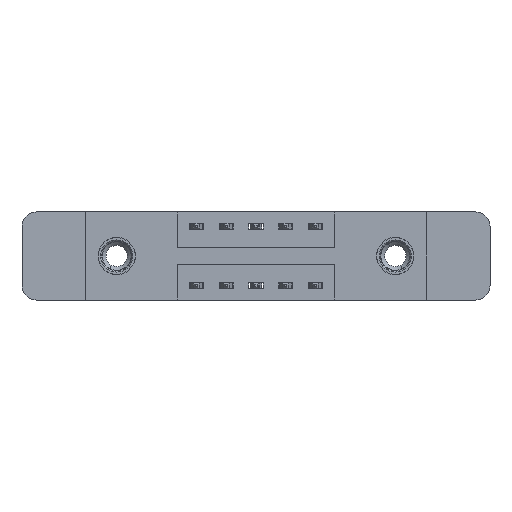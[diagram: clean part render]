
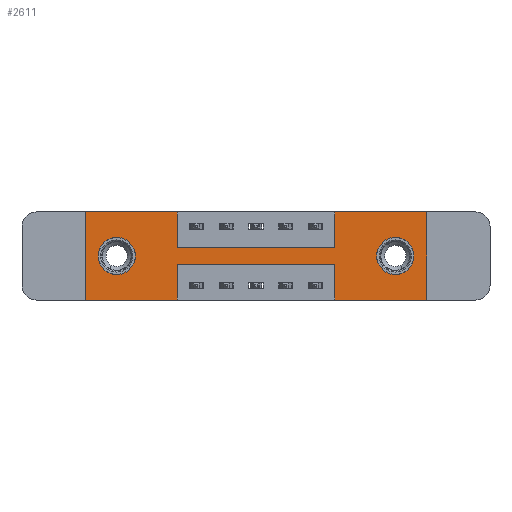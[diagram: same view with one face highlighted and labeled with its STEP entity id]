
A CAD part, front view. The second image highlights one B-rep face of the part: STEP entity #2611.
In plain terms, the highlighted planar face has unit normal (0, -1, 0).
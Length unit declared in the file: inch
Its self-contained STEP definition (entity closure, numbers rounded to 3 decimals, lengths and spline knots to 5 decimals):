
#114 = CARTESIAN_POINT ( 'NONE',  ( 1.0475, 0., 0. ) ) ;
#251 = CIRCLE ( 'NONE', #4269, 0.078 ) ;
#421 = VERTEX_POINT ( 'NONE', #11232 ) ;
#464 = EDGE_LOOP ( 'NONE', ( #4634, #6377, #11064, #1808, #10592, #12197, #609, #7411, #11130, #10439, #12892, #6052 ) ) ;
#492 = AXIS2_PLACEMENT_3D ( 'NONE', #10237, #594, #2548 ) ;
#591 = CARTESIAN_POINT ( 'NONE',  ( 1.3025, 0., -0.185 ) ) ;
#594 = DIRECTION ( 'NONE',  ( 0., 1., 0. ) ) ;
#609 = ORIENTED_EDGE ( 'NONE', *, *, #4410, .F. ) ;
#617 = VECTOR ( 'NONE', #7813, 39.37008 ) ;
#828 = CARTESIAN_POINT ( 'NONE',  ( 1.0475, 0., 0. ) ) ;
#1084 = VERTEX_POINT ( 'NONE', #4495 ) ;
#1183 = DIRECTION ( 'NONE',  ( 0., 0., -1. ) ) ;
#1267 = VECTOR ( 'NONE', #8334, 39.37008 ) ;
#1575 = DIRECTION ( 'NONE',  ( 0., 1., 0. ) ) ;
#1769 = VECTOR ( 'NONE', #8291, 39.37008 ) ;
#1782 = CARTESIAN_POINT ( 'NONE',  ( 0., 0., 0. ) ) ;
#1808 = ORIENTED_EDGE ( 'NONE', *, *, #2719, .F. ) ;
#1887 = VERTEX_POINT ( 'NONE', #10619 ) ;
#1908 = EDGE_CURVE ( 'NONE', #3533, #421, #5184, .T. ) ;
#1961 = CARTESIAN_POINT ( 'NONE',  ( 0., 0., 0. ) ) ;
#2085 = CARTESIAN_POINT ( 'NONE',  ( 0.3875, 0., -0.22 ) ) ;
#2548 = DIRECTION ( 'NONE',  ( 0., 0., -1. ) ) ;
#2595 = FACE_BOUND ( 'NONE', #10058, .T. ) ;
#2611 = ADVANCED_FACE ( 'NONE', ( #5841, #2595, #8096 ), #9073, .T. ) ;
#2719 = EDGE_CURVE ( 'NONE', #1887, #12294, #10290, .T. ) ;
#2818 = VECTOR ( 'NONE', #5249, 39.37008 ) ;
#2833 = DIRECTION ( 'NONE',  ( 1., 0., 0. ) ) ;
#3062 = VERTEX_POINT ( 'NONE', #9270 ) ;
#3256 = CIRCLE ( 'NONE', #3486, 0.078 ) ;
#3486 = AXIS2_PLACEMENT_3D ( 'NONE', #9402, #10741, #7279 ) ;
#3509 = EDGE_CURVE ( 'NONE', #6834, #1887, #9177, .T. ) ;
#3533 = VERTEX_POINT ( 'NONE', #4042 ) ;
#3568 = LINE ( 'NONE', #10120, #11354 ) ;
#3586 = CARTESIAN_POINT ( 'NONE',  ( 0., 0., -0.37 ) ) ;
#3628 = CARTESIAN_POINT ( 'NONE',  ( 1.435, 0., 0. ) ) ;
#3706 = VECTOR ( 'NONE', #5077, 39.37008 ) ;
#3946 = VERTEX_POINT ( 'NONE', #11497 ) ;
#4042 = CARTESIAN_POINT ( 'NONE',  ( 0., 0., 0. ) ) ;
#4269 = AXIS2_PLACEMENT_3D ( 'NONE', #12480, #6275, #10357 ) ;
#4318 = VERTEX_POINT ( 'NONE', #4919 ) ;
#4410 = EDGE_CURVE ( 'NONE', #7584, #10257, #6044, .T. ) ;
#4495 = CARTESIAN_POINT ( 'NONE',  ( 0.1325, 0., -0.263 ) ) ;
#4504 = CARTESIAN_POINT ( 'NONE',  ( 0., 0., -0.37 ) ) ;
#4634 = ORIENTED_EDGE ( 'NONE', *, *, #8993, .F. ) ;
#4919 = CARTESIAN_POINT ( 'NONE',  ( 0.1325, 0., -0.107 ) ) ;
#5027 = CARTESIAN_POINT ( 'NONE',  ( 0.3875, 0., -0.15 ) ) ;
#5077 = DIRECTION ( 'NONE',  ( -1., 0., 0. ) ) ;
#5184 = LINE ( 'NONE', #1961, #2818 ) ;
#5249 = DIRECTION ( 'NONE',  ( 1., 0., 0. ) ) ;
#5359 = ORIENTED_EDGE ( 'NONE', *, *, #10028, .T. ) ;
#5434 = VECTOR ( 'NONE', #2833, 39.37008 ) ;
#5790 = VERTEX_POINT ( 'NONE', #10631 ) ;
#5841 = FACE_BOUND ( 'NONE', #7109, .T. ) ;
#6044 = LINE ( 'NONE', #828, #6667 ) ;
#6052 = ORIENTED_EDGE ( 'NONE', *, *, #12785, .F. ) ;
#6210 = DIRECTION ( 'NONE',  ( 1., 0., 0. ) ) ;
#6275 = DIRECTION ( 'NONE',  ( 0., 1., 0. ) ) ;
#6377 = ORIENTED_EDGE ( 'NONE', *, *, #8666, .F. ) ;
#6405 = CIRCLE ( 'NONE', #9101, 0.078 ) ;
#6555 = CIRCLE ( 'NONE', #492, 0.078 ) ;
#6667 = VECTOR ( 'NONE', #10342, 39.37008 ) ;
#6746 = CARTESIAN_POINT ( 'NONE',  ( 1.3025, 0., -0.263 ) ) ;
#6834 = VERTEX_POINT ( 'NONE', #3628 ) ;
#7109 = EDGE_LOOP ( 'NONE', ( #12772, #7836 ) ) ;
#7142 = LINE ( 'NONE', #12775, #1267 ) ;
#7279 = DIRECTION ( 'NONE',  ( 0., 0., 1. ) ) ;
#7411 = ORIENTED_EDGE ( 'NONE', *, *, #11434, .F. ) ;
#7571 = CARTESIAN_POINT ( 'NONE',  ( 0.3875, 0., -0.15 ) ) ;
#7584 = VERTEX_POINT ( 'NONE', #10205 ) ;
#7674 = VECTOR ( 'NONE', #6210, 39.37008 ) ;
#7813 = DIRECTION ( 'NONE',  ( 0., 0., 1. ) ) ;
#7836 = ORIENTED_EDGE ( 'NONE', *, *, #11478, .T. ) ;
#8092 = CARTESIAN_POINT ( 'NONE',  ( 1.0475, 0., -0.37 ) ) ;
#8096 = FACE_OUTER_BOUND ( 'NONE', #464, .T. ) ;
#8291 = DIRECTION ( 'NONE',  ( -1., 0., 0. ) ) ;
#8315 = EDGE_CURVE ( 'NONE', #421, #11276, #12032, .T. ) ;
#8334 = DIRECTION ( 'NONE',  ( 0., 0., -1. ) ) ;
#8666 = EDGE_CURVE ( 'NONE', #3062, #13025, #11742, .T. ) ;
#8861 = CARTESIAN_POINT ( 'NONE',  ( 1.0475, 0., -0.37 ) ) ;
#8870 = AXIS2_PLACEMENT_3D ( 'NONE', #3586, #11061, #13369 ) ;
#8993 = EDGE_CURVE ( 'NONE', #13025, #5790, #7142, .T. ) ;
#9073 = PLANE ( 'NONE',  #8870 ) ;
#9101 = AXIS2_PLACEMENT_3D ( 'NONE', #591, #1575, #11297 ) ;
#9177 = LINE ( 'NONE', #10327, #12541 ) ;
#9188 = DIRECTION ( 'NONE',  ( -1., 0., 0. ) ) ;
#9270 = CARTESIAN_POINT ( 'NONE',  ( 1.0475, 0., -0.22 ) ) ;
#9402 = CARTESIAN_POINT ( 'NONE',  ( 0.1325, 0., -0.185 ) ) ;
#9445 = EDGE_CURVE ( 'NONE', #10505, #3533, #9766, .T. ) ;
#9492 = VERTEX_POINT ( 'NONE', #6746 ) ;
#9766 = LINE ( 'NONE', #13140, #617 ) ;
#10028 = EDGE_CURVE ( 'NONE', #4318, #1084, #3256, .T. ) ;
#10058 = EDGE_LOOP ( 'NONE', ( #5359, #12626 ) ) ;
#10061 = LINE ( 'NONE', #8861, #12391 ) ;
#10120 = CARTESIAN_POINT ( 'NONE',  ( 0., 0., -0.37 ) ) ;
#10205 = CARTESIAN_POINT ( 'NONE',  ( 1.0475, 0., -0.15 ) ) ;
#10237 = CARTESIAN_POINT ( 'NONE',  ( 1.3025, 0., -0.185 ) ) ;
#10257 = VERTEX_POINT ( 'NONE', #114 ) ;
#10290 = LINE ( 'NONE', #13514, #3706 ) ;
#10327 = CARTESIAN_POINT ( 'NONE',  ( 1.435, 0., 0. ) ) ;
#10342 = DIRECTION ( 'NONE',  ( 0., 0., 1. ) ) ;
#10343 = EDGE_CURVE ( 'NONE', #3946, #9492, #6405, .T. ) ;
#10357 = DIRECTION ( 'NONE',  ( 0., 0., 1. ) ) ;
#10439 = ORIENTED_EDGE ( 'NONE', *, *, #1908, .F. ) ;
#10505 = VERTEX_POINT ( 'NONE', #4504 ) ;
#10592 = ORIENTED_EDGE ( 'NONE', *, *, #3509, .F. ) ;
#10619 = CARTESIAN_POINT ( 'NONE',  ( 1.435, 0., -0.37 ) ) ;
#10631 = CARTESIAN_POINT ( 'NONE',  ( 0.3875, 0., -0.37 ) ) ;
#10741 = DIRECTION ( 'NONE',  ( 0., 1., 0. ) ) ;
#10780 = EDGE_CURVE ( 'NONE', #10257, #6834, #11565, .T. ) ;
#10791 = EDGE_CURVE ( 'NONE', #1084, #4318, #251, .T. ) ;
#10887 = CARTESIAN_POINT ( 'NONE',  ( 0.3875, 0., -0.22 ) ) ;
#10979 = CARTESIAN_POINT ( 'NONE',  ( 0.3875, 0., 0. ) ) ;
#11029 = EDGE_CURVE ( 'NONE', #12294, #3062, #10061, .T. ) ;
#11061 = DIRECTION ( 'NONE',  ( 0., -1., 0. ) ) ;
#11064 = ORIENTED_EDGE ( 'NONE', *, *, #11029, .F. ) ;
#11130 = ORIENTED_EDGE ( 'NONE', *, *, #8315, .F. ) ;
#11232 = CARTESIAN_POINT ( 'NONE',  ( 0.3875, 0., 0. ) ) ;
#11276 = VERTEX_POINT ( 'NONE', #7571 ) ;
#11297 = DIRECTION ( 'NONE',  ( 0., 0., -1. ) ) ;
#11354 = VECTOR ( 'NONE', #9188, 39.37008 ) ;
#11434 = EDGE_CURVE ( 'NONE', #11276, #7584, #12426, .T. ) ;
#11478 = EDGE_CURVE ( 'NONE', #9492, #3946, #6555, .T. ) ;
#11497 = CARTESIAN_POINT ( 'NONE',  ( 1.3025, 0., -0.107 ) ) ;
#11565 = LINE ( 'NONE', #1782, #7674 ) ;
#11742 = LINE ( 'NONE', #2085, #1769 ) ;
#12032 = LINE ( 'NONE', #10979, #12560 ) ;
#12197 = ORIENTED_EDGE ( 'NONE', *, *, #10780, .F. ) ;
#12246 = DIRECTION ( 'NONE',  ( 0., 0., 1. ) ) ;
#12294 = VERTEX_POINT ( 'NONE', #8092 ) ;
#12391 = VECTOR ( 'NONE', #12246, 39.37008 ) ;
#12426 = LINE ( 'NONE', #5027, #5434 ) ;
#12480 = CARTESIAN_POINT ( 'NONE',  ( 0.1325, 0., -0.185 ) ) ;
#12541 = VECTOR ( 'NONE', #13479, 39.37008 ) ;
#12560 = VECTOR ( 'NONE', #1183, 39.37008 ) ;
#12626 = ORIENTED_EDGE ( 'NONE', *, *, #10791, .T. ) ;
#12772 = ORIENTED_EDGE ( 'NONE', *, *, #10343, .T. ) ;
#12775 = CARTESIAN_POINT ( 'NONE',  ( 0.3875, 0., -0.37 ) ) ;
#12785 = EDGE_CURVE ( 'NONE', #5790, #10505, #3568, .T. ) ;
#12892 = ORIENTED_EDGE ( 'NONE', *, *, #9445, .F. ) ;
#13025 = VERTEX_POINT ( 'NONE', #10887 ) ;
#13140 = CARTESIAN_POINT ( 'NONE',  ( 0., 0., 0. ) ) ;
#13369 = DIRECTION ( 'NONE',  ( 0., 0., -1. ) ) ;
#13479 = DIRECTION ( 'NONE',  ( 0., 0., -1. ) ) ;
#13514 = CARTESIAN_POINT ( 'NONE',  ( 0., 0., -0.37 ) ) ;
